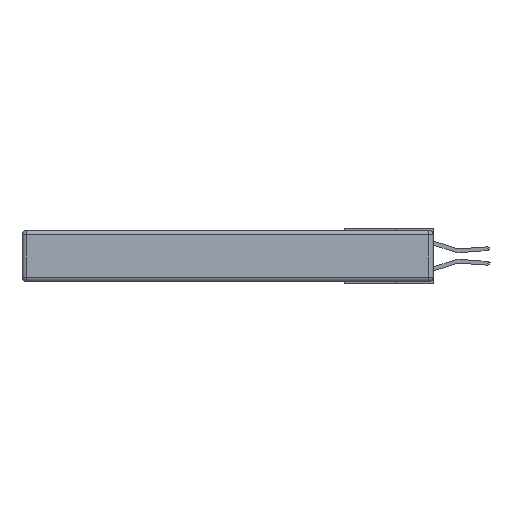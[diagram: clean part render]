
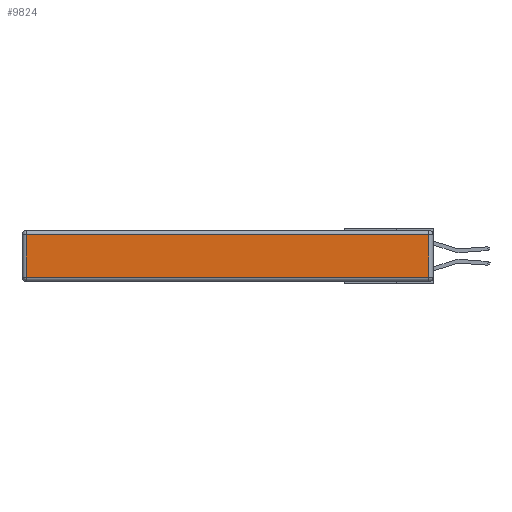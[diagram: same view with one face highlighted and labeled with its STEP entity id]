
A CAD part, left-side view. The second image highlights one B-rep face of the part: STEP entity #9824.
In plain terms, the highlighted planar face has unit normal (-1, 0, 0).
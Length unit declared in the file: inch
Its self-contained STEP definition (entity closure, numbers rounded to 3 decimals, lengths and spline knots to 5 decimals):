
#127 = ORIENTED_EDGE ( 'NONE', *, *, #1046, .T. ) ;
#267 = CARTESIAN_POINT ( 'NONE',  ( 0., 2.72, -0.03 ) ) ;
#800 = VERTEX_POINT ( 'NONE', #3679 ) ;
#1046 = EDGE_CURVE ( 'NONE', #8557, #5197, #10633, .T. ) ;
#1727 = AXIS2_PLACEMENT_3D ( 'NONE', #8367, #10671, #14209 ) ;
#2251 = EDGE_CURVE ( 'NONE', #800, #8557, #10776, .T. ) ;
#2328 = PLANE ( 'NONE',  #1727 ) ;
#3679 = CARTESIAN_POINT ( 'NONE',  ( 0., 0.03, -0.03 ) ) ;
#4196 = DIRECTION ( 'NONE',  ( 0., 0., -1. ) ) ;
#4745 = VECTOR ( 'NONE', #9366, 39.37008 ) ;
#5197 = VERTEX_POINT ( 'NONE', #9998 ) ;
#5228 = ORIENTED_EDGE ( 'NONE', *, *, #2251, .T. ) ;
#5840 = ORIENTED_EDGE ( 'NONE', *, *, #6543, .T. ) ;
#6543 = EDGE_CURVE ( 'NONE', #5197, #11910, #7604, .T. ) ;
#7224 = DIRECTION ( 'NONE',  ( 0., 1., 0. ) ) ;
#7604 = LINE ( 'NONE', #13260, #10404 ) ;
#8044 = EDGE_LOOP ( 'NONE', ( #5840, #14167, #5228, #127 ) ) ;
#8284 = LINE ( 'NONE', #15237, #4745 ) ;
#8348 = VECTOR ( 'NONE', #7224, 39.37008 ) ;
#8367 = CARTESIAN_POINT ( 'NONE',  ( 0., 0., -0.343 ) ) ;
#8450 = DIRECTION ( 'NONE',  ( 0., -1., 0. ) ) ;
#8557 = VERTEX_POINT ( 'NONE', #267 ) ;
#9366 = DIRECTION ( 'NONE',  ( 0., 0., 1. ) ) ;
#9495 = VECTOR ( 'NONE', #4196, 39.37008 ) ;
#9518 = CARTESIAN_POINT ( 'NONE',  ( 0., 2.75, -0.03 ) ) ;
#9824 = ADVANCED_FACE ( 'NONE', ( #10022 ), #2328, .T. ) ;
#9998 = CARTESIAN_POINT ( 'NONE',  ( 0., 2.72, -0.313 ) ) ;
#10022 = FACE_OUTER_BOUND ( 'NONE', #8044, .T. ) ;
#10404 = VECTOR ( 'NONE', #8450, 39.37008 ) ;
#10633 = LINE ( 'NONE', #11447, #9495 ) ;
#10671 = DIRECTION ( 'NONE',  ( -1., 0., 0. ) ) ;
#10776 = LINE ( 'NONE', #9518, #8348 ) ;
#11447 = CARTESIAN_POINT ( 'NONE',  ( 0., 2.72, -0.343 ) ) ;
#11560 = EDGE_CURVE ( 'NONE', #11910, #800, #8284, .T. ) ;
#11910 = VERTEX_POINT ( 'NONE', #12014 ) ;
#12014 = CARTESIAN_POINT ( 'NONE',  ( 0., 0.03, -0.313 ) ) ;
#13260 = CARTESIAN_POINT ( 'NONE',  ( 0., 0., -0.313 ) ) ;
#14167 = ORIENTED_EDGE ( 'NONE', *, *, #11560, .T. ) ;
#14209 = DIRECTION ( 'NONE',  ( 0., 0., 1. ) ) ;
#15237 = CARTESIAN_POINT ( 'NONE',  ( 0., 0.03, -0.343 ) ) ;
